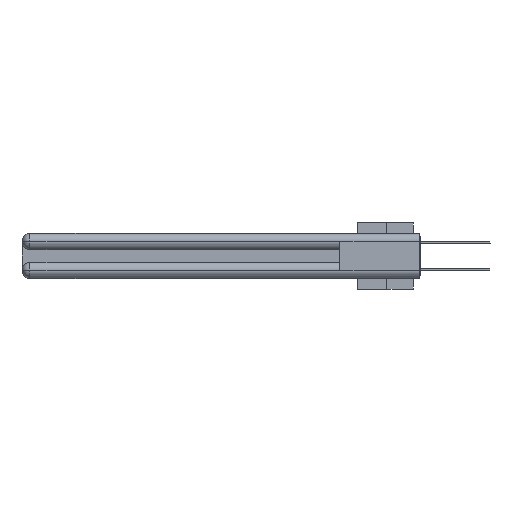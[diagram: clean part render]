
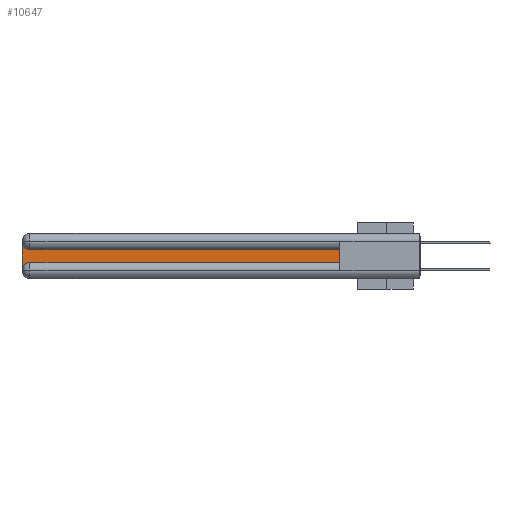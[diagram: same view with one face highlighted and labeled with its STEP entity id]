
A CAD part, left-side view. The second image highlights one B-rep face of the part: STEP entity #10647.
In plain terms, the highlighted planar face has unit normal (-1, 0, 0).
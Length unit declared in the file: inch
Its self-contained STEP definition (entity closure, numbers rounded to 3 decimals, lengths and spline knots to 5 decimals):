
#875 = VERTEX_POINT ( 'NONE', #35023 ) ;
#2078 = DIRECTION ( 'NONE',  ( 1., 0., 0. ) ) ;
#2182 = VERTEX_POINT ( 'NONE', #26591 ) ;
#3775 = ORIENTED_EDGE ( 'NONE', *, *, #25243, .T. ) ;
#5329 = VECTOR ( 'NONE', #16046, 39.37008 ) ;
#6170 = VERTEX_POINT ( 'NONE', #30726 ) ;
#7018 = ORIENTED_EDGE ( 'NONE', *, *, #7262, .T. ) ;
#7033 = DIRECTION ( 'NONE',  ( 1., 0., 0. ) ) ;
#7262 = EDGE_CURVE ( 'NONE', #17745, #875, #18231, .T. ) ;
#8226 = ORIENTED_EDGE ( 'NONE', *, *, #20702, .T. ) ;
#10516 = ORIENTED_EDGE ( 'NONE', *, *, #34761, .T. ) ;
#10647 = ADVANCED_FACE ( 'NONE', ( #31374 ), #13283, .F. ) ;
#11132 = EDGE_CURVE ( 'NONE', #875, #2182, #35359, .T. ) ;
#11255 = VERTEX_POINT ( 'NONE', #31215 ) ;
#11587 = DIRECTION ( 'NONE',  ( 1., 0., 0. ) ) ;
#11803 = VERTEX_POINT ( 'NONE', #36674 ) ;
#11817 = AXIS2_PLACEMENT_3D ( 'NONE', #30840, #2078, #36323 ) ;
#12262 = EDGE_CURVE ( 'NONE', #2182, #11255, #21036, .T. ) ;
#12745 = DIRECTION ( 'NONE',  ( 0., 0., -1. ) ) ;
#13283 = PLANE ( 'NONE',  #11817 ) ;
#14221 = CARTESIAN_POINT ( 'NONE',  ( 0.075, 2.94, -0.0625 ) ) ;
#15092 = DIRECTION ( 'NONE',  ( 0., 0., 1. ) ) ;
#16046 = DIRECTION ( 'NONE',  ( 0., 0., -1. ) ) ;
#17677 = AXIS2_PLACEMENT_3D ( 'NONE', #29939, #7033, #12745 ) ;
#17692 = DIRECTION ( 'NONE',  ( 0., -1., 0. ) ) ;
#17745 = VERTEX_POINT ( 'NONE', #34363 ) ;
#18231 = LINE ( 'NONE', #20727, #30687 ) ;
#20702 = EDGE_CURVE ( 'NONE', #11803, #17745, #24036, .T. ) ;
#20727 = CARTESIAN_POINT ( 'NONE',  ( 0.075, 0.6, -0.2175 ) ) ;
#21036 = CIRCLE ( 'NONE', #32170, 0.06 ) ;
#21464 = CARTESIAN_POINT ( 'NONE',  ( 0.075, 3., -0.2175 ) ) ;
#23113 = ORIENTED_EDGE ( 'NONE', *, *, #12262, .T. ) ;
#23790 = CARTESIAN_POINT ( 'NONE',  ( 0.075, 0.6, -0.2175 ) ) ;
#24036 = LINE ( 'NONE', #23790, #28517 ) ;
#25243 = EDGE_CURVE ( 'NONE', #11255, #6170, #25339, .T. ) ;
#25339 = LINE ( 'NONE', #21464, #5329 ) ;
#26591 = CARTESIAN_POINT ( 'NONE',  ( 0.075, 2.94, -0.1225 ) ) ;
#26997 = CARTESIAN_POINT ( 'NONE',  ( 0.075, 0.6, -0.1225 ) ) ;
#28517 = VECTOR ( 'NONE', #17692, 39.37008 ) ;
#29939 = CARTESIAN_POINT ( 'NONE',  ( 0.075, 2.94, -0.2775 ) ) ;
#30687 = VECTOR ( 'NONE', #15092, 39.37008 ) ;
#30726 = CARTESIAN_POINT ( 'NONE',  ( 0.075, 3., -0.2775 ) ) ;
#30840 = CARTESIAN_POINT ( 'NONE',  ( 0.075, 3., -0.1225 ) ) ;
#31215 = CARTESIAN_POINT ( 'NONE',  ( 0.075, 3., -0.0625 ) ) ;
#31340 = VECTOR ( 'NONE', #35603, 39.37008 ) ;
#31374 = FACE_OUTER_BOUND ( 'NONE', #35804, .T. ) ;
#31397 = DIRECTION ( 'NONE',  ( 0., 0., -1. ) ) ;
#32170 = AXIS2_PLACEMENT_3D ( 'NONE', #14221, #11587, #31397 ) ;
#32427 = ORIENTED_EDGE ( 'NONE', *, *, #11132, .T. ) ;
#34363 = CARTESIAN_POINT ( 'NONE',  ( 0.075, 0.6, -0.2175 ) ) ;
#34379 = CIRCLE ( 'NONE', #17677, 0.06 ) ;
#34761 = EDGE_CURVE ( 'NONE', #6170, #11803, #34379, .T. ) ;
#35023 = CARTESIAN_POINT ( 'NONE',  ( 0.075, 0.6, -0.1225 ) ) ;
#35359 = LINE ( 'NONE', #26997, #31340 ) ;
#35603 = DIRECTION ( 'NONE',  ( 0., 1., 0. ) ) ;
#35804 = EDGE_LOOP ( 'NONE', ( #32427, #23113, #3775, #10516, #8226, #7018 ) ) ;
#36323 = DIRECTION ( 'NONE',  ( 0., 0., -1. ) ) ;
#36674 = CARTESIAN_POINT ( 'NONE',  ( 0.075, 2.94, -0.2175 ) ) ;
